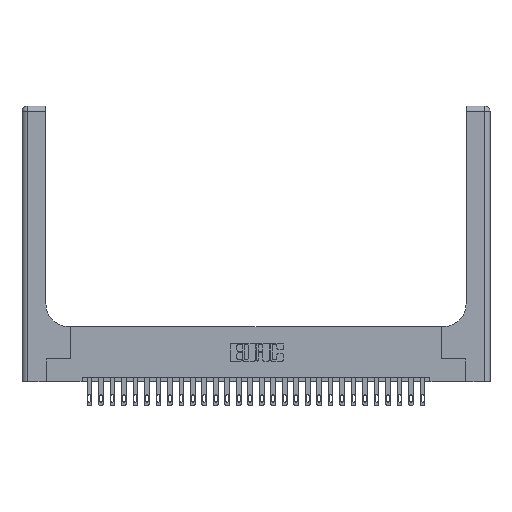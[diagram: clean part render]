
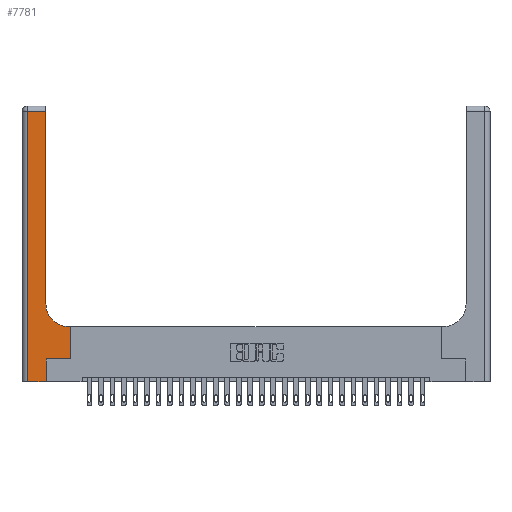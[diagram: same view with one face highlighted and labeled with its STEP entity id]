
A CAD part, top view. The second image highlights one B-rep face of the part: STEP entity #7781.
In plain terms, the highlighted planar face has unit normal (0, 0, 1).
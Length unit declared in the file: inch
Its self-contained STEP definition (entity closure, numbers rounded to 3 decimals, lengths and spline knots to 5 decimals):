
#215 = AXIS2_PLACEMENT_3D ( 'NONE', #22752, #12466, #20586 ) ;
#487 = LINE ( 'NONE', #17255, #15233 ) ;
#506 = ORIENTED_EDGE ( 'NONE', *, *, #6151, .T. ) ;
#703 = EDGE_LOOP ( 'NONE', ( #10395, #13826, #14774, #9831, #11088, #506, #21566, #22962, #1447 ) ) ;
#951 = VERTEX_POINT ( 'NONE', #6115 ) ;
#1447 = ORIENTED_EDGE ( 'NONE', *, *, #20489, .T. ) ;
#1735 = CARTESIAN_POINT ( 'NONE',  ( 0.528, 0.6, 0.37 ) ) ;
#1803 = VERTEX_POINT ( 'NONE', #1735 ) ;
#1850 = LINE ( 'NONE', #14150, #20684 ) ;
#1962 = CARTESIAN_POINT ( 'NONE',  ( 0., 0., 0.37 ) ) ;
#2206 = CARTESIAN_POINT ( 'NONE',  ( 0.265, 0.25, 0.37 ) ) ;
#2511 = VECTOR ( 'NONE', #20389, 39.37008 ) ;
#3443 = CARTESIAN_POINT ( 'NONE',  ( 0.06, 0., 0.37 ) ) ;
#3757 = DIRECTION ( 'NONE',  ( -1., 0., 0. ) ) ;
#5342 = EDGE_CURVE ( 'NONE', #1803, #7216, #16507, .T. ) ;
#5629 = LINE ( 'NONE', #13878, #6422 ) ;
#5909 = EDGE_CURVE ( 'NONE', #951, #23861, #5629, .T. ) ;
#5935 = EDGE_CURVE ( 'NONE', #17168, #1803, #1850, .T. ) ;
#6115 = CARTESIAN_POINT ( 'NONE',  ( 0.265, 0., 0.37 ) ) ;
#6151 = EDGE_CURVE ( 'NONE', #23861, #17168, #23878, .T. ) ;
#6363 = VECTOR ( 'NONE', #21875, 39.37008 ) ;
#6422 = VECTOR ( 'NONE', #7921, 39.37008 ) ;
#6498 = VECTOR ( 'NONE', #24709, 39.37008 ) ;
#7216 = VERTEX_POINT ( 'NONE', #11558 ) ;
#7406 = EDGE_CURVE ( 'NONE', #11069, #951, #14260, .T. ) ;
#7489 = CARTESIAN_POINT ( 'NONE',  ( 0.265, 0.25, 0.37 ) ) ;
#7781 = ADVANCED_FACE ( 'NONE', ( #12553 ), #20405, .F. ) ;
#7921 = DIRECTION ( 'NONE',  ( 0., 1., 0. ) ) ;
#8233 = CARTESIAN_POINT ( 'NONE',  ( 0.26, 0.85, 0.37 ) ) ;
#8865 = VERTEX_POINT ( 'NONE', #15291 ) ;
#9165 = CARTESIAN_POINT ( 'NONE',  ( 0.06, 3., 0.37 ) ) ;
#9831 = ORIENTED_EDGE ( 'NONE', *, *, #7406, .T. ) ;
#10071 = CARTESIAN_POINT ( 'NONE',  ( 0.06, 2.94, 0.37 ) ) ;
#10381 = VERTEX_POINT ( 'NONE', #8233 ) ;
#10395 = ORIENTED_EDGE ( 'NONE', *, *, #21454, .T. ) ;
#11069 = VERTEX_POINT ( 'NONE', #3443 ) ;
#11088 = ORIENTED_EDGE ( 'NONE', *, *, #5909, .T. ) ;
#11558 = CARTESIAN_POINT ( 'NONE',  ( 0.51, 0.6, 0.37 ) ) ;
#11854 = LINE ( 'NONE', #24321, #2511 ) ;
#12466 = DIRECTION ( 'NONE',  ( 0., 0., -1. ) ) ;
#12553 = FACE_OUTER_BOUND ( 'NONE', #703, .T. ) ;
#12977 = VERTEX_POINT ( 'NONE', #10071 ) ;
#13826 = ORIENTED_EDGE ( 'NONE', *, *, #19341, .T. ) ;
#13878 = CARTESIAN_POINT ( 'NONE',  ( 0.265, 0., 0.37 ) ) ;
#14150 = CARTESIAN_POINT ( 'NONE',  ( 0.528, 0.25, 0.37 ) ) ;
#14260 = LINE ( 'NONE', #1962, #6498 ) ;
#14774 = ORIENTED_EDGE ( 'NONE', *, *, #21302, .T. ) ;
#15233 = VECTOR ( 'NONE', #23605, 39.37008 ) ;
#15291 = CARTESIAN_POINT ( 'NONE',  ( 0.26, 2.94, 0.37 ) ) ;
#16480 = AXIS2_PLACEMENT_3D ( 'NONE', #24759, #18787, #3757 ) ;
#16507 = LINE ( 'NONE', #26396, #21495 ) ;
#17168 = VERTEX_POINT ( 'NONE', #17189 ) ;
#17189 = CARTESIAN_POINT ( 'NONE',  ( 0.528, 0.25, 0.37 ) ) ;
#17255 = CARTESIAN_POINT ( 'NONE',  ( 0., 2.94, 0.37 ) ) ;
#17260 = DIRECTION ( 'NONE',  ( 1., 0., 0. ) ) ;
#18787 = DIRECTION ( 'NONE',  ( 0., 0., -1. ) ) ;
#19341 = EDGE_CURVE ( 'NONE', #8865, #12977, #487, .T. ) ;
#19581 = LINE ( 'NONE', #9165, #6363 ) ;
#20389 = DIRECTION ( 'NONE',  ( 0., 1., 0. ) ) ;
#20405 = PLANE ( 'NONE',  #16480 ) ;
#20489 = EDGE_CURVE ( 'NONE', #7216, #10381, #20519, .T. ) ;
#20519 = CIRCLE ( 'NONE', #215, 0.25 ) ;
#20586 = DIRECTION ( 'NONE',  ( 1., 0., 0. ) ) ;
#20684 = VECTOR ( 'NONE', #22140, 39.37008 ) ;
#21302 = EDGE_CURVE ( 'NONE', #12977, #11069, #19581, .T. ) ;
#21454 = EDGE_CURVE ( 'NONE', #10381, #8865, #11854, .T. ) ;
#21495 = VECTOR ( 'NONE', #22441, 39.37008 ) ;
#21566 = ORIENTED_EDGE ( 'NONE', *, *, #5935, .T. ) ;
#21875 = DIRECTION ( 'NONE',  ( 0., -1., 0. ) ) ;
#22140 = DIRECTION ( 'NONE',  ( 0., 1., 0. ) ) ;
#22441 = DIRECTION ( 'NONE',  ( -1., 0., 0. ) ) ;
#22752 = CARTESIAN_POINT ( 'NONE',  ( 0.51, 0.85, 0.37 ) ) ;
#22962 = ORIENTED_EDGE ( 'NONE', *, *, #5342, .T. ) ;
#23605 = DIRECTION ( 'NONE',  ( -1., 0., 0. ) ) ;
#23861 = VERTEX_POINT ( 'NONE', #2206 ) ;
#23878 = LINE ( 'NONE', #7489, #25888 ) ;
#24321 = CARTESIAN_POINT ( 'NONE',  ( 0.26, 3., 0.37 ) ) ;
#24709 = DIRECTION ( 'NONE',  ( 1., 0., 0. ) ) ;
#24759 = CARTESIAN_POINT ( 'NONE',  ( 0., 3., 0.37 ) ) ;
#25888 = VECTOR ( 'NONE', #17260, 39.37008 ) ;
#26396 = CARTESIAN_POINT ( 'NONE',  ( 0.26, 0.6, 0.37 ) ) ;
